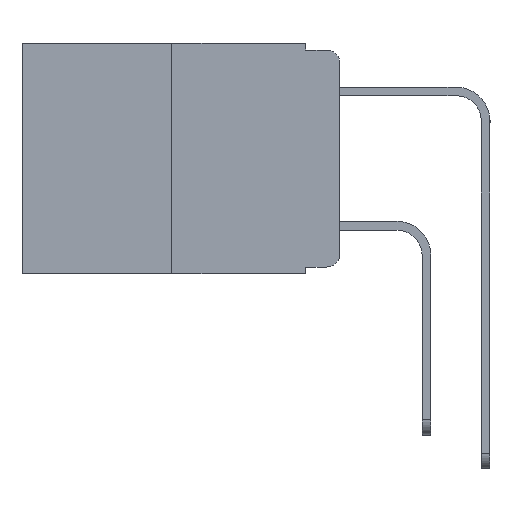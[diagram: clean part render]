
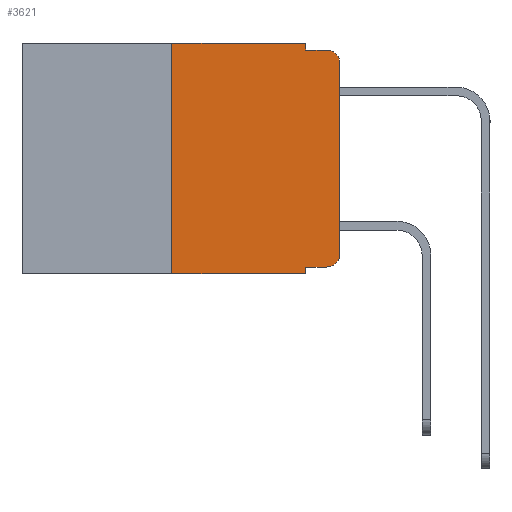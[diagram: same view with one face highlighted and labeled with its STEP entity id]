
A CAD part, left-side view. The second image highlights one B-rep face of the part: STEP entity #3621.
In plain terms, the highlighted planar face has unit normal (-1, 0, 0).
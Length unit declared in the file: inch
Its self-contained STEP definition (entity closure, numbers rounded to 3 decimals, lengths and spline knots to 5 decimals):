
#237 = DIRECTION ( 'NONE',  ( 0., 0., -1. ) ) ;
#445 = DIRECTION ( 'NONE',  ( 0., -1., 0. ) ) ;
#1120 = LINE ( 'NONE', #21766, #10926 ) ;
#1640 = AXIS2_PLACEMENT_3D ( 'NONE', #14394, #14101, #14098 ) ;
#1833 = VECTOR ( 'NONE', #15603, 39.37008 ) ;
#2189 = VERTEX_POINT ( 'NONE', #13677 ) ;
#2224 = EDGE_CURVE ( 'NONE', #9931, #2189, #10936, .T. ) ;
#2400 = LINE ( 'NONE', #12268, #19893 ) ;
#3193 = DIRECTION ( 'NONE',  ( 0., 0., -1. ) ) ;
#3403 = EDGE_CURVE ( 'NONE', #7299, #9931, #20746, .T. ) ;
#3621 = ADVANCED_FACE ( 'NONE', ( #11647 ), #14653, .F. ) ;
#3812 = VERTEX_POINT ( 'NONE', #12048 ) ;
#4046 = CARTESIAN_POINT ( 'NONE',  ( 0., 0.02, -0.333 ) ) ;
#4098 = LINE ( 'NONE', #20866, #12638 ) ;
#4597 = EDGE_CURVE ( 'NONE', #7299, #10039, #7628, .T. ) ;
#4946 = EDGE_LOOP ( 'NONE', ( #14103, #18545, #19045, #10708, #7260, #16201, #8873, #13335, #9941, #10449 ) ) ;
#5360 = CARTESIAN_POINT ( 'NONE',  ( 0., 0.473, -0.343 ) ) ;
#5763 = EDGE_CURVE ( 'NONE', #9715, #18645, #6538, .T. ) ;
#6538 = LINE ( 'NONE', #13915, #1833 ) ;
#6571 = DIRECTION ( 'NONE',  ( 0., 0., 1. ) ) ;
#6926 = EDGE_CURVE ( 'NONE', #19603, #15224, #1120, .T. ) ;
#6971 = LINE ( 'NONE', #5360, #19805 ) ;
#7096 = VECTOR ( 'NONE', #7177, 39.37008 ) ;
#7163 = DIRECTION ( 'NONE',  ( 0., -1., 0. ) ) ;
#7177 = DIRECTION ( 'NONE',  ( 0., 0., -1. ) ) ;
#7260 = ORIENTED_EDGE ( 'NONE', *, *, #9808, .F. ) ;
#7299 = VERTEX_POINT ( 'NONE', #19376 ) ;
#7628 = LINE ( 'NONE', #12214, #7096 ) ;
#7951 = DIRECTION ( 'NONE',  ( 1., 0., 0. ) ) ;
#8490 = CARTESIAN_POINT ( 'NONE',  ( 0., 0., -0.03 ) ) ;
#8537 = CARTESIAN_POINT ( 'NONE',  ( 0., 0.051, -0.333 ) ) ;
#8873 = ORIENTED_EDGE ( 'NONE', *, *, #18855, .T. ) ;
#9218 = EDGE_CURVE ( 'NONE', #15224, #3812, #4098, .T. ) ;
#9715 = VERTEX_POINT ( 'NONE', #20334 ) ;
#9808 = EDGE_CURVE ( 'NONE', #18645, #19603, #2400, .T. ) ;
#9931 = VERTEX_POINT ( 'NONE', #4046 ) ;
#9937 = CARTESIAN_POINT ( 'NONE',  ( 0., 0., 0. ) ) ;
#9941 = ORIENTED_EDGE ( 'NONE', *, *, #3403, .T. ) ;
#10039 = VERTEX_POINT ( 'NONE', #17868 ) ;
#10343 = EDGE_CURVE ( 'NONE', #19825, #3812, #17564, .T. ) ;
#10449 = ORIENTED_EDGE ( 'NONE', *, *, #2224, .T. ) ;
#10706 = DIRECTION ( 'NONE',  ( -1., 0., 0. ) ) ;
#10708 = ORIENTED_EDGE ( 'NONE', *, *, #6926, .F. ) ;
#10926 = VECTOR ( 'NONE', #3193, 39.37008 ) ;
#10936 = CIRCLE ( 'NONE', #1640, 0.02 ) ;
#11478 = EDGE_CURVE ( 'NONE', #2189, #19825, #13858, .T. ) ;
#11647 = FACE_OUTER_BOUND ( 'NONE', #4946, .T. ) ;
#11918 = VECTOR ( 'NONE', #16502, 39.37008 ) ;
#12048 = CARTESIAN_POINT ( 'NONE',  ( 0., 0.02, -0.01 ) ) ;
#12214 = CARTESIAN_POINT ( 'NONE',  ( 0., 0.051, 0. ) ) ;
#12231 = AXIS2_PLACEMENT_3D ( 'NONE', #17917, #7951, #19646 ) ;
#12268 = CARTESIAN_POINT ( 'NONE',  ( 0., 0.473, 0. ) ) ;
#12638 = VECTOR ( 'NONE', #445, 39.37008 ) ;
#13335 = ORIENTED_EDGE ( 'NONE', *, *, #4597, .F. ) ;
#13351 = VECTOR ( 'NONE', #6571, 39.37008 ) ;
#13677 = CARTESIAN_POINT ( 'NONE',  ( 0., 0., -0.313 ) ) ;
#13809 = DIRECTION ( 'NONE',  ( 0., -1., 0. ) ) ;
#13858 = LINE ( 'NONE', #9937, #13351 ) ;
#13915 = CARTESIAN_POINT ( 'NONE',  ( 0., 0.25, 0. ) ) ;
#14098 = DIRECTION ( 'NONE',  ( 0., 0., -1. ) ) ;
#14101 = DIRECTION ( 'NONE',  ( -1., 0., 0. ) ) ;
#14103 = ORIENTED_EDGE ( 'NONE', *, *, #11478, .T. ) ;
#14394 = CARTESIAN_POINT ( 'NONE',  ( 0., 0.02, -0.313 ) ) ;
#14653 = PLANE ( 'NONE',  #12231 ) ;
#15224 = VERTEX_POINT ( 'NONE', #17408 ) ;
#15603 = DIRECTION ( 'NONE',  ( 0., 0., 1. ) ) ;
#15683 = CARTESIAN_POINT ( 'NONE',  ( 0., 0.051, 0. ) ) ;
#16201 = ORIENTED_EDGE ( 'NONE', *, *, #5763, .F. ) ;
#16502 = DIRECTION ( 'NONE',  ( 0., -1., 0. ) ) ;
#17408 = CARTESIAN_POINT ( 'NONE',  ( 0., 0.051, -0.01 ) ) ;
#17564 = CIRCLE ( 'NONE', #19418, 0.02 ) ;
#17868 = CARTESIAN_POINT ( 'NONE',  ( 0., 0.051, -0.343 ) ) ;
#17917 = CARTESIAN_POINT ( 'NONE',  ( 0., 0.473, 0. ) ) ;
#18219 = CARTESIAN_POINT ( 'NONE',  ( 0., 0.25, 0. ) ) ;
#18545 = ORIENTED_EDGE ( 'NONE', *, *, #10343, .T. ) ;
#18645 = VERTEX_POINT ( 'NONE', #18219 ) ;
#18855 = EDGE_CURVE ( 'NONE', #9715, #10039, #6971, .T. ) ;
#19045 = ORIENTED_EDGE ( 'NONE', *, *, #9218, .F. ) ;
#19376 = CARTESIAN_POINT ( 'NONE',  ( 0., 0.051, -0.333 ) ) ;
#19418 = AXIS2_PLACEMENT_3D ( 'NONE', #20659, #10706, #237 ) ;
#19603 = VERTEX_POINT ( 'NONE', #15683 ) ;
#19646 = DIRECTION ( 'NONE',  ( 0., 0., -1. ) ) ;
#19805 = VECTOR ( 'NONE', #13809, 39.37008 ) ;
#19825 = VERTEX_POINT ( 'NONE', #8490 ) ;
#19893 = VECTOR ( 'NONE', #7163, 39.37008 ) ;
#20334 = CARTESIAN_POINT ( 'NONE',  ( 0., 0.25, -0.343 ) ) ;
#20659 = CARTESIAN_POINT ( 'NONE',  ( 0., 0.02, -0.03 ) ) ;
#20746 = LINE ( 'NONE', #8537, #11918 ) ;
#20866 = CARTESIAN_POINT ( 'NONE',  ( 0., 0.051, -0.01 ) ) ;
#21766 = CARTESIAN_POINT ( 'NONE',  ( 0., 0.051, 0. ) ) ;
